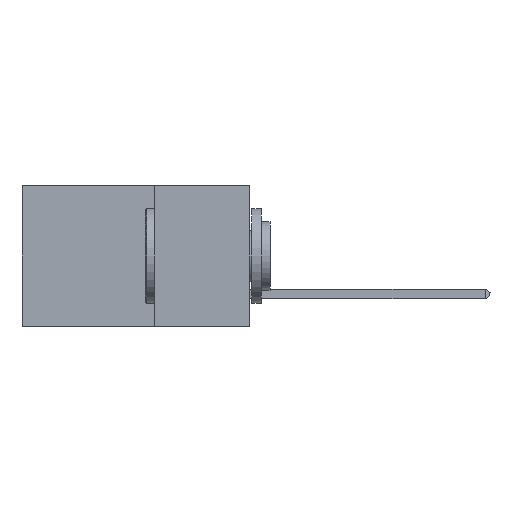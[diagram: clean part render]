
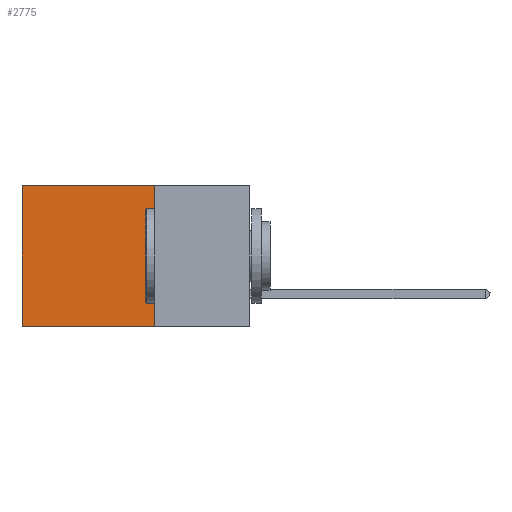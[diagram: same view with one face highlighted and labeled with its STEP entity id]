
A CAD part, left-side view. The second image highlights one B-rep face of the part: STEP entity #2775.
In plain terms, the highlighted planar face has unit normal (-1, 0, 0).
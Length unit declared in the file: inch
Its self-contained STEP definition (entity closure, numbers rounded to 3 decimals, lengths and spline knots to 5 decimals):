
#1532 = CARTESIAN_POINT ( 'NONE',  ( 0.2875, 0.25, 0. ) ) ;
#2119 = DIRECTION ( 'NONE',  ( 0., 0., -1. ) ) ;
#2775 = ADVANCED_FACE ( 'NONE', ( #29136 ), #9092, .F. ) ;
#5470 = ORIENTED_EDGE ( 'NONE', *, *, #20717, .T. ) ;
#6530 = ORIENTED_EDGE ( 'NONE', *, *, #27904, .F. ) ;
#6709 = ORIENTED_EDGE ( 'NONE', *, *, #33525, .T. ) ;
#6920 = CARTESIAN_POINT ( 'NONE',  ( 0.2875, 0.6, 0. ) ) ;
#9092 = PLANE ( 'NONE',  #28354 ) ;
#9390 = VERTEX_POINT ( 'NONE', #6920 ) ;
#9717 = VECTOR ( 'NONE', #20723, 39.37008 ) ;
#10306 = ORIENTED_EDGE ( 'NONE', *, *, #17243, .F. ) ;
#13249 = CARTESIAN_POINT ( 'NONE',  ( 0.2875, 0.25, 0. ) ) ;
#14700 = CARTESIAN_POINT ( 'NONE',  ( 0.2875, 0.25, 0. ) ) ;
#15783 = DIRECTION ( 'NONE',  ( 0., 0., -1. ) ) ;
#16394 = CARTESIAN_POINT ( 'NONE',  ( 0.2875, 0.6, -0.37 ) ) ;
#17243 = EDGE_CURVE ( 'NONE', #26848, #19042, #18683, .T. ) ;
#18683 = LINE ( 'NONE', #1532, #9717 ) ;
#19042 = VERTEX_POINT ( 'NONE', #25442 ) ;
#20717 = EDGE_CURVE ( 'NONE', #26848, #9390, #32103, .T. ) ;
#20723 = DIRECTION ( 'NONE',  ( 0., 0., -1. ) ) ;
#20854 = EDGE_LOOP ( 'NONE', ( #6709, #6530, #10306, #5470 ) ) ;
#22666 = VERTEX_POINT ( 'NONE', #16394 ) ;
#22823 = VECTOR ( 'NONE', #2119, 39.37008 ) ;
#23037 = DIRECTION ( 'NONE',  ( 0., 1., 0. ) ) ;
#23179 = VECTOR ( 'NONE', #26772, 39.37008 ) ;
#25029 = CARTESIAN_POINT ( 'NONE',  ( 0.2875, 0.25, 0. ) ) ;
#25442 = CARTESIAN_POINT ( 'NONE',  ( 0.2875, 0.25, -0.37 ) ) ;
#26565 = CARTESIAN_POINT ( 'NONE',  ( 0.2875, 0.6, 0. ) ) ;
#26772 = DIRECTION ( 'NONE',  ( 0., 1., 0. ) ) ;
#26848 = VERTEX_POINT ( 'NONE', #25029 ) ;
#27042 = LINE ( 'NONE', #26565, #22823 ) ;
#27129 = CARTESIAN_POINT ( 'NONE',  ( 0.2875, 0.25, -0.37 ) ) ;
#27904 = EDGE_CURVE ( 'NONE', #19042, #22666, #32584, .T. ) ;
#28354 = AXIS2_PLACEMENT_3D ( 'NONE', #13249, #32500, #15783 ) ;
#28727 = VECTOR ( 'NONE', #23037, 39.37008 ) ;
#29136 = FACE_OUTER_BOUND ( 'NONE', #20854, .T. ) ;
#32103 = LINE ( 'NONE', #14700, #28727 ) ;
#32500 = DIRECTION ( 'NONE',  ( 1., 0., 0. ) ) ;
#32584 = LINE ( 'NONE', #27129, #23179 ) ;
#33525 = EDGE_CURVE ( 'NONE', #9390, #22666, #27042, .T. ) ;
